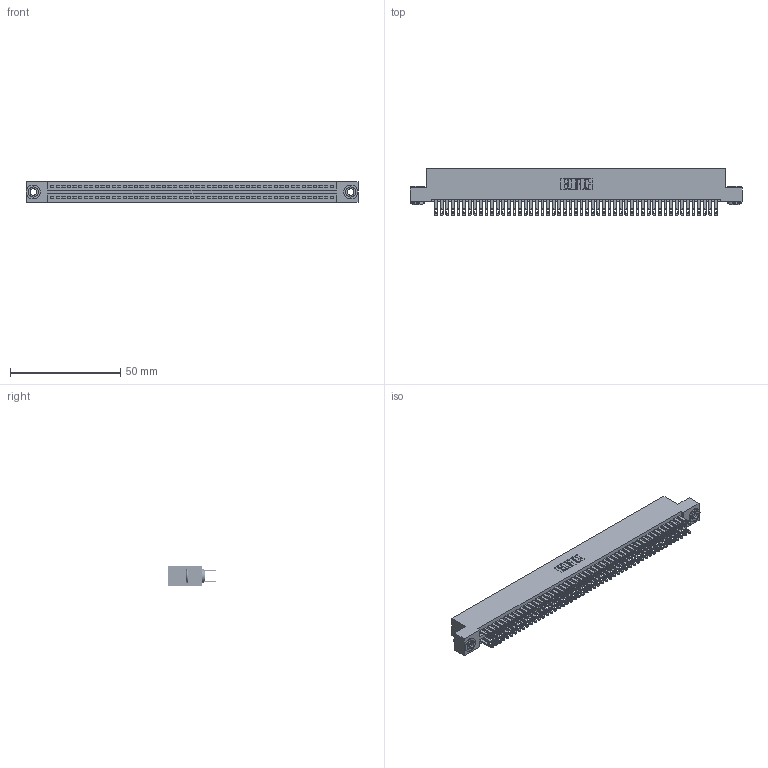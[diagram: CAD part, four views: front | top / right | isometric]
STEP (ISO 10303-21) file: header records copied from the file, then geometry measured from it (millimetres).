
FILE_DESCRIPTION (( 'STEP AP203' ), '1' );
FILE_NAME ('345-102-500-203.STEP', '2018-10-05T18:20:11', ( '' ), ( '' ), 'SwSTEP 2.0', 'SolidWorks 2016', '' );
FILE_SCHEMA (( 'CONFIG_CONTROL_DESIGN' ));
Length unit declared in the file: inch
Products named in the file (4): 345-292-001_345-293-100; 345 Part_Flush Mounting Lugs - 0.156 Dia-TH; 345-102-500-203; 345-250-002_345-250-002-102
Assembly tree (105 placements, depth 2):
  345-102-500-203
    345 Part_Flush Mounting Lugs - 0.156 Dia-TH
    345-292-001_345-293-100  x102
    345-250-002_345-250-002-102  x2
Bounding box: 150.75 x 21.51 x 9.4 mm (x, y, z)
Volume: 15058.5 mm3; surface area: 23678.6 mm2
Topology: 105 solids, 105 shells, 4856 faces, 14799 edges, 9862 vertices
Faces by surface type: plane 2844, cylinder 2004, cone 8
Entity records: 39384 total; most frequent: CARTESIAN_POINT 6567, ORIENTED_EDGE 6494, DIRECTION 5813, EDGE_CURVE 3247, LINE 2883, VECTOR 2883, VERTEX_POINT 2162, AXIS2_PLACEMENT_3D 1465
